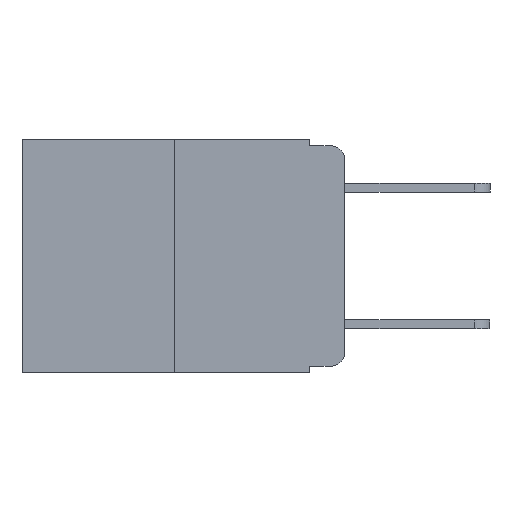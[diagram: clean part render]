
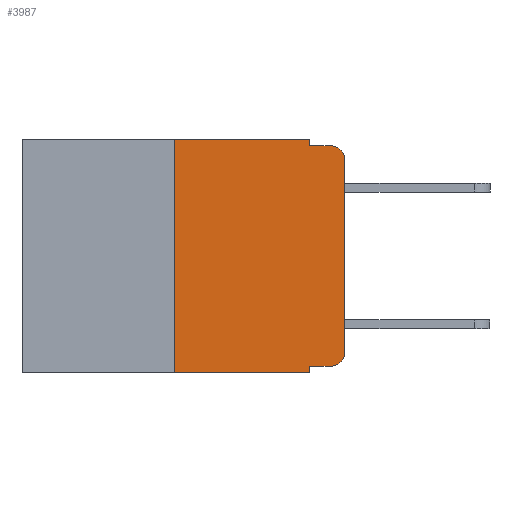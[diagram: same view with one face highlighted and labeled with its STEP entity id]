
A CAD part, left-side view. The second image highlights one B-rep face of the part: STEP entity #3987.
In plain terms, the highlighted planar face has unit normal (-1, 0, 0).
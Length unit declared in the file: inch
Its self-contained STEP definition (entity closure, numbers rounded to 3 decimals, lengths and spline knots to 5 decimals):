
#390 = VERTEX_POINT ( 'NONE', #8843 ) ;
#1158 = AXIS2_PLACEMENT_3D ( 'NONE', #5861, #12284, #6998 ) ;
#1230 = LINE ( 'NONE', #9876, #9561 ) ;
#1298 = ORIENTED_EDGE ( 'NONE', *, *, #7140, .F. ) ;
#1338 = DIRECTION ( 'NONE',  ( 0., 0., -1. ) ) ;
#1437 = CARTESIAN_POINT ( 'NONE',  ( 0., 0.25, 0. ) ) ;
#1470 = CARTESIAN_POINT ( 'NONE',  ( 0., 0.473, 0. ) ) ;
#1523 = ORIENTED_EDGE ( 'NONE', *, *, #7145, .F. ) ;
#1576 = VECTOR ( 'NONE', #9950, 39.37008 ) ;
#1943 = VECTOR ( 'NONE', #11487, 39.37008 ) ;
#2003 = CARTESIAN_POINT ( 'NONE',  ( 0., 0.25, -0.343 ) ) ;
#2356 = AXIS2_PLACEMENT_3D ( 'NONE', #5829, #12266, #6973 ) ;
#2599 = DIRECTION ( 'NONE',  ( 0., -1., 0. ) ) ;
#2681 = LINE ( 'NONE', #1470, #12634 ) ;
#3201 = ORIENTED_EDGE ( 'NONE', *, *, #7123, .F. ) ;
#3451 = CARTESIAN_POINT ( 'NONE',  ( 0., 0.02, -0.333 ) ) ;
#3500 = CARTESIAN_POINT ( 'NONE',  ( 0., 0.051, 0. ) ) ;
#3987 = ADVANCED_FACE ( 'NONE', ( #6994 ), #9040, .F. ) ;
#4014 = VERTEX_POINT ( 'NONE', #12329 ) ;
#4064 = VERTEX_POINT ( 'NONE', #11696 ) ;
#4454 = CARTESIAN_POINT ( 'NONE',  ( 0., 0.051, -0.333 ) ) ;
#4460 = VERTEX_POINT ( 'NONE', #8556 ) ;
#4492 = VERTEX_POINT ( 'NONE', #2003 ) ;
#4558 = VECTOR ( 'NONE', #7014, 39.37008 ) ;
#4680 = CARTESIAN_POINT ( 'NONE',  ( 0., 0.051, 0. ) ) ;
#4936 = CIRCLE ( 'NONE', #12622, 0.02 ) ;
#5160 = VERTEX_POINT ( 'NONE', #5461 ) ;
#5461 = CARTESIAN_POINT ( 'NONE',  ( 0., 0.02, -0.01 ) ) ;
#5556 = ORIENTED_EDGE ( 'NONE', *, *, #6909, .T. ) ;
#5763 = CARTESIAN_POINT ( 'NONE',  ( 0., 0.02, -0.03 ) ) ;
#5829 = CARTESIAN_POINT ( 'NONE',  ( 0., 0.473, 0. ) ) ;
#5851 = ORIENTED_EDGE ( 'NONE', *, *, #7160, .F. ) ;
#5861 = CARTESIAN_POINT ( 'NONE',  ( 0., 0.02, -0.313 ) ) ;
#6144 = VERTEX_POINT ( 'NONE', #11979 ) ;
#6208 = CARTESIAN_POINT ( 'NONE',  ( 0., 0.473, -0.343 ) ) ;
#6322 = EDGE_CURVE ( 'NONE', #7419, #4014, #2681, .T. ) ;
#6901 = DIRECTION ( 'NONE',  ( 0., 0., -1. ) ) ;
#6909 = EDGE_CURVE ( 'NONE', #4492, #4460, #12740, .T. ) ;
#6973 = DIRECTION ( 'NONE',  ( 0., 0., -1. ) ) ;
#6994 = FACE_OUTER_BOUND ( 'NONE', #10393, .T. ) ;
#6998 = DIRECTION ( 'NONE',  ( 0., 0., -1. ) ) ;
#7014 = DIRECTION ( 'NONE',  ( 0., 0., 1. ) ) ;
#7116 = EDGE_CURVE ( 'NONE', #4064, #390, #7207, .T. ) ;
#7119 = EDGE_CURVE ( 'NONE', #390, #5160, #4936, .T. ) ;
#7123 = EDGE_CURVE ( 'NONE', #6144, #5160, #1230, .T. ) ;
#7140 = EDGE_CURVE ( 'NONE', #4014, #6144, #12314, .T. ) ;
#7145 = EDGE_CURVE ( 'NONE', #4492, #7419, #10111, .T. ) ;
#7160 = EDGE_CURVE ( 'NONE', #7295, #4460, #11900, .T. ) ;
#7161 = EDGE_CURVE ( 'NONE', #7295, #8559, #12141, .T. ) ;
#7162 = EDGE_CURVE ( 'NONE', #8559, #4064, #7194, .T. ) ;
#7194 = CIRCLE ( 'NONE', #1158, 0.02 ) ;
#7207 = LINE ( 'NONE', #7930, #4558 ) ;
#7295 = VERTEX_POINT ( 'NONE', #4454 ) ;
#7419 = VERTEX_POINT ( 'NONE', #1437 ) ;
#7536 = VECTOR ( 'NONE', #7980, 39.37008 ) ;
#7566 = ORIENTED_EDGE ( 'NONE', *, *, #7161, .T. ) ;
#7930 = CARTESIAN_POINT ( 'NONE',  ( 0., 0., 0. ) ) ;
#7980 = DIRECTION ( 'NONE',  ( 0., 0., 1. ) ) ;
#8556 = CARTESIAN_POINT ( 'NONE',  ( 0., 0.051, -0.343 ) ) ;
#8559 = VERTEX_POINT ( 'NONE', #3451 ) ;
#8754 = ORIENTED_EDGE ( 'NONE', *, *, #7162, .T. ) ;
#8843 = CARTESIAN_POINT ( 'NONE',  ( 0., 0., -0.03 ) ) ;
#8986 = DIRECTION ( 'NONE',  ( 0., -1., 0. ) ) ;
#9040 = PLANE ( 'NONE',  #2356 ) ;
#9060 = CARTESIAN_POINT ( 'NONE',  ( 0., 0.051, -0.333 ) ) ;
#9327 = ORIENTED_EDGE ( 'NONE', *, *, #7116, .T. ) ;
#9331 = DIRECTION ( 'NONE',  ( 0., -1., 0. ) ) ;
#9561 = VECTOR ( 'NONE', #8986, 39.37008 ) ;
#9832 = VECTOR ( 'NONE', #1338, 39.37008 ) ;
#9876 = CARTESIAN_POINT ( 'NONE',  ( 0., 0.051, -0.01 ) ) ;
#9910 = CARTESIAN_POINT ( 'NONE',  ( 0., 0.25, 0. ) ) ;
#9950 = DIRECTION ( 'NONE',  ( 0., -1., 0. ) ) ;
#10111 = LINE ( 'NONE', #9910, #7536 ) ;
#10393 = EDGE_LOOP ( 'NONE', ( #9327, #12549, #3201, #1298, #11470, #1523, #5556, #5851, #7566, #8754 ) ) ;
#11470 = ORIENTED_EDGE ( 'NONE', *, *, #6322, .F. ) ;
#11487 = DIRECTION ( 'NONE',  ( 0., 0., -1. ) ) ;
#11696 = CARTESIAN_POINT ( 'NONE',  ( 0., 0., -0.313 ) ) ;
#11900 = LINE ( 'NONE', #3500, #9832 ) ;
#11979 = CARTESIAN_POINT ( 'NONE',  ( 0., 0.051, -0.01 ) ) ;
#12141 = LINE ( 'NONE', #9060, #1576 ) ;
#12216 = DIRECTION ( 'NONE',  ( -1., 0., 0. ) ) ;
#12266 = DIRECTION ( 'NONE',  ( 1., 0., 0. ) ) ;
#12284 = DIRECTION ( 'NONE',  ( -1., 0., 0. ) ) ;
#12314 = LINE ( 'NONE', #4680, #1943 ) ;
#12329 = CARTESIAN_POINT ( 'NONE',  ( 0., 0.051, 0. ) ) ;
#12507 = VECTOR ( 'NONE', #9331, 39.37008 ) ;
#12549 = ORIENTED_EDGE ( 'NONE', *, *, #7119, .T. ) ;
#12622 = AXIS2_PLACEMENT_3D ( 'NONE', #5763, #12216, #6901 ) ;
#12634 = VECTOR ( 'NONE', #2599, 39.37008 ) ;
#12740 = LINE ( 'NONE', #6208, #12507 ) ;
